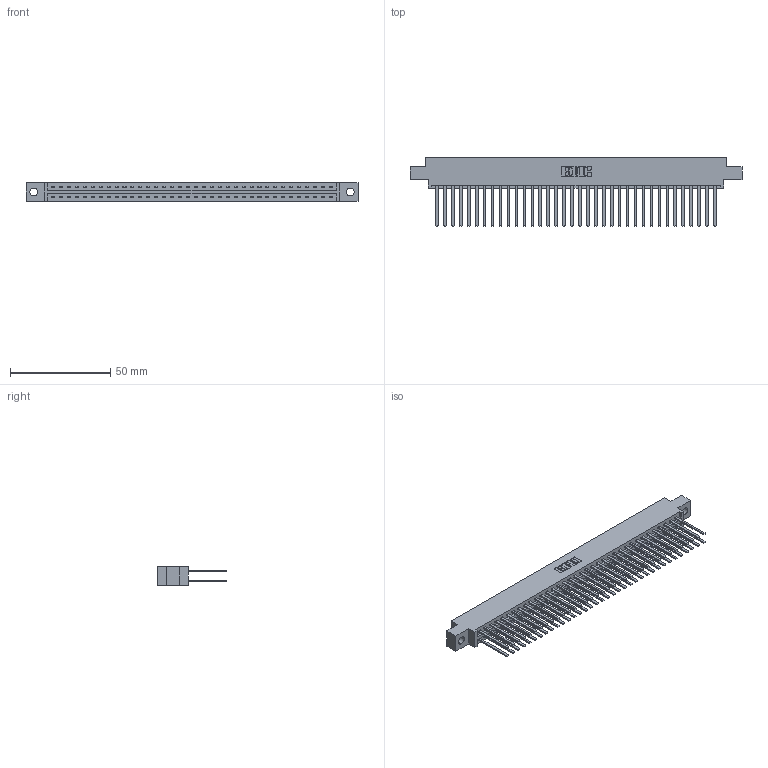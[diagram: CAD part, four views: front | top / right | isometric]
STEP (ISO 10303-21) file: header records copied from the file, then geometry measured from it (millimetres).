
FILE_DESCRIPTION (( 'STEP AP203' ), '1' );
FILE_NAME ('337-072-544-804.STEP', '2019-10-15T11:49:14', ( '' ), ( '' ), 'SwSTEP 2.0', 'SolidWorks 2016', '' );
FILE_SCHEMA (( 'CONFIG_CONTROL_DESIGN' ));
Length unit declared in the file: inch
Products named in the file (3): 345-292-001_345-293-144; 337-072-544-804; 337 Part_0.170 Offset - 0.156 Dia-TH
Assembly tree (73 placements, depth 2):
  337-072-544-804
    337 Part_0.170 Offset - 0.156 Dia-TH
    345-292-001_345-293-144  x72
Bounding box: 165.66 x 34.3 x 9.4 mm (x, y, z)
Volume: 18182.5 mm3; surface area: 23699.5 mm2
Topology: 73 solids, 73 shells, 3574 faces, 10619 edges, 6982 vertices
Faces by surface type: plane 2522, cylinder 1052
Entity records: 28639 total; most frequent: CARTESIAN_POINT 4830, ORIENTED_EDGE 4766, DIRECTION 4115, EDGE_CURVE 2383, LINE 2259, VECTOR 2259, VERTEX_POINT 1586, AXIS2_PLACEMENT_3D 928
